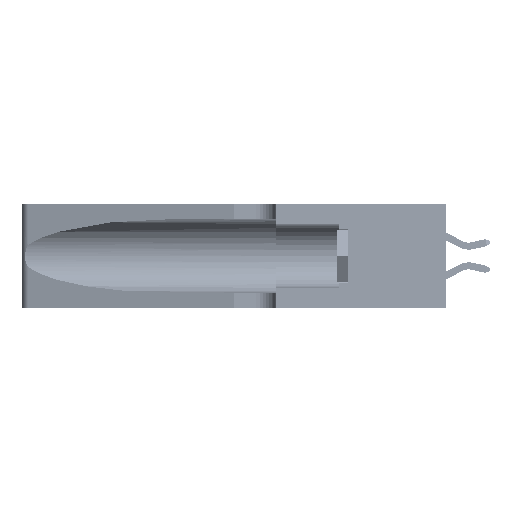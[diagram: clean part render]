
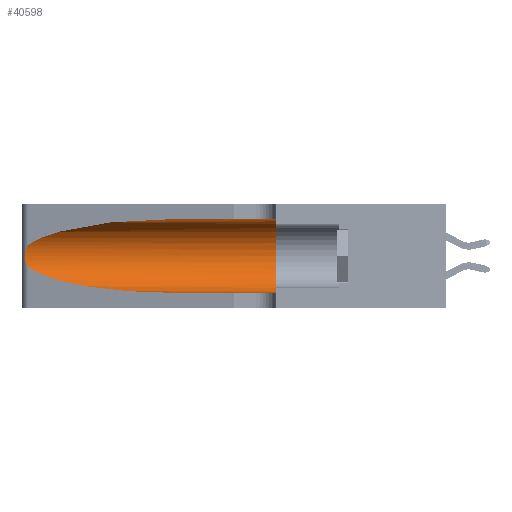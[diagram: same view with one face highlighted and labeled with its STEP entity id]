
A CAD part, left-side view. The second image highlights one B-rep face of the part: STEP entity #40598.
In plain terms, the highlighted cylindrical face has radius 3.308 mm (diameter 6.617 mm), a partial arc.
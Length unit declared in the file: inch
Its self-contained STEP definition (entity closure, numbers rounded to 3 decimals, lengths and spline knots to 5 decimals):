
#165 = CARTESIAN_POINT ( 'NONE',  ( 0.2373, 1.15595, 0.08982 ) ) ;
#395 = CARTESIAN_POINT ( 'NONE',  ( 0.1305, 1.61858, 0.185 ) ) ;
#1396 = CARTESIAN_POINT ( 'NONE',  ( 0.26018, 1.23835, 0.19895 ) ) ;
#1444 = ORIENTED_EDGE ( 'NONE', *, *, #46868, .T. ) ;
#2937 = ORIENTED_EDGE ( 'NONE', *, *, #30242, .T. ) ;
#3268 = DIRECTION ( 'NONE',  ( 0., 0., 1. ) ) ;
#3982 = CYLINDRICAL_SURFACE ( 'NONE', #19545, 0.13025 ) ;
#4039 = VECTOR ( 'NONE', #16669, 39.37008 ) ;
#4175 = CARTESIAN_POINT ( 'NONE',  ( 0.18966, 0.96281, 0.05475 ) ) ;
#4848 = CARTESIAN_POINT ( 'NONE',  ( 0.1305, 0.72297, 0.31525 ) ) ;
#5222 = FACE_OUTER_BOUND ( 'NONE', #39873, .T. ) ;
#5376 = CARTESIAN_POINT ( 'NONE',  ( 0.26075, 1.23896, 0.178 ) ) ;
#6524 = EDGE_CURVE ( 'NONE', #23491, #16954, #32752, .T. ) ;
#7786 = CARTESIAN_POINT ( 'NONE',  ( 0.1305, 0.35, 0.05475 ) ) ;
#8304 = DIRECTION ( 'NONE',  ( 0., 0., -1. ) ) ;
#8749 = CARTESIAN_POINT ( 'NONE',  ( 0.2373, 1.15595, 0.28018 ) ) ;
#9259 = CARTESIAN_POINT ( 'NONE',  ( 0.25856, 1.23593, 0.16098 ) ) ;
#10930 = VERTEX_POINT ( 'NONE', #28211 ) ;
#13111 = CARTESIAN_POINT ( 'NONE',  ( 0.25639, 1.23186, 0.15144 ) ) ;
#13795 = VERTEX_POINT ( 'NONE', #40203 ) ;
#14588 = CARTESIAN_POINT ( 'NONE',  ( 0.1305, 1.61858, 0.31525 ) ) ;
#16669 = DIRECTION ( 'NONE',  ( 0., -1., 0. ) ) ;
#16732 = CARTESIAN_POINT ( 'NONE',  ( 0.25487, 1.22718, 0.22369 ) ) ;
#16888 = CARTESIAN_POINT ( 'NONE',  ( 0.25487, 1.22718, 0.14631 ) ) ;
#16954 = VERTEX_POINT ( 'NONE', #48494 ) ;
#18870 = B_SPLINE_CURVE_WITH_KNOTS ( 'NONE', 3,
 ( #16732, #35430, #20499, #46677, #24292, #1396, #28073, #5376, #31846, #9259, #35581, #13111, #39286, #16888 ),
 .UNSPECIFIED., .F., .F.,
 ( 4, 2, 2, 2, 2, 2, 4 ),
 ( 0., 0.00027, 0.00053, 0.00107, 0.0016, 0.00187, 0.00214 ),
 .UNSPECIFIED. ) ;
#19545 = AXIS2_PLACEMENT_3D ( 'NONE', #395, #30924, #8304 ) ;
#20499 = CARTESIAN_POINT ( 'NONE',  ( 0.25639, 1.23184, 0.21858 ) ) ;
#21071 = EDGE_CURVE ( 'NONE', #10930, #13795, #48585, .T. ) ;
#22062 = CIRCLE ( 'NONE', #25625, 0.13025 ) ;
#22507 =( BOUNDED_CURVE ( )  B_SPLINE_CURVE ( 3, ( #4848, #27566, #8749, #35082 ),
 .UNSPECIFIED., .F., .T. ) 
 B_SPLINE_CURVE_WITH_KNOTS ( ( 4, 4 ),
 ( 1.5708, 2.84003 ),
 .UNSPECIFIED. ) 
 CURVE ( )  GEOMETRIC_REPRESENTATION_ITEM ( )  RATIONAL_B_SPLINE_CURVE ( ( 1., 0.87, 0.87, 1. ) ) 
 REPRESENTATION_ITEM ( '' )  );
#22757 = VECTOR ( 'NONE', #48307, 39.37008 ) ;
#23143 = CARTESIAN_POINT ( 'NONE',  ( 0.25487, 1.22718, 0.14631 ) ) ;
#23491 = VERTEX_POINT ( 'NONE', #43228 ) ;
#24292 = CARTESIAN_POINT ( 'NONE',  ( 0.25854, 1.2359, 0.20912 ) ) ;
#25625 = AXIS2_PLACEMENT_3D ( 'NONE', #48428, #26029, #3268 ) ;
#26029 = DIRECTION ( 'NONE',  ( 0., 1., 0. ) ) ;
#27566 = CARTESIAN_POINT ( 'NONE',  ( 0.18966, 0.96281, 0.31525 ) ) ;
#28073 = CARTESIAN_POINT ( 'NONE',  ( 0.26075, 1.23896, 0.19203 ) ) ;
#28211 = CARTESIAN_POINT ( 'NONE',  ( 0.25487, 1.22718, 0.14631 ) ) ;
#28576 = ORIENTED_EDGE ( 'NONE', *, *, #36854, .T. ) ;
#30242 = EDGE_CURVE ( 'NONE', #23491, #42915, #22507, .T. ) ;
#30719 = CARTESIAN_POINT ( 'NONE',  ( 0.1305, 0.72297, 0.05475 ) ) ;
#30924 = DIRECTION ( 'NONE',  ( 0., -1., 0. ) ) ;
#31126 = ORIENTED_EDGE ( 'NONE', *, *, #6524, .F. ) ;
#31192 = ORIENTED_EDGE ( 'NONE', *, *, #34451, .F. ) ;
#31846 = CARTESIAN_POINT ( 'NONE',  ( 0.26017, 1.23833, 0.17102 ) ) ;
#32752 = LINE ( 'NONE', #14588, #22757 ) ;
#34246 = LINE ( 'NONE', #42839, #4039 ) ;
#34451 = EDGE_CURVE ( 'NONE', #16954, #42503, #22062, .T. ) ;
#35082 = CARTESIAN_POINT ( 'NONE',  ( 0.25487, 1.22718, 0.22369 ) ) ;
#35430 = CARTESIAN_POINT ( 'NONE',  ( 0.25555, 1.22994, 0.2215 ) ) ;
#35581 = CARTESIAN_POINT ( 'NONE',  ( 0.25789, 1.23486, 0.15765 ) ) ;
#36425 = CARTESIAN_POINT ( 'NONE',  ( 0.25487, 1.22718, 0.22369 ) ) ;
#36854 = EDGE_CURVE ( 'NONE', #13795, #42503, #34246, .T. ) ;
#38516 = ORIENTED_EDGE ( 'NONE', *, *, #21071, .T. ) ;
#39286 = CARTESIAN_POINT ( 'NONE',  ( 0.25555, 1.22993, 0.14849 ) ) ;
#39873 = EDGE_LOOP ( 'NONE', ( #2937, #1444, #38516, #28576, #31192, #31126 ) ) ;
#40203 = CARTESIAN_POINT ( 'NONE',  ( 0.1305, 0.72297, 0.05475 ) ) ;
#40598 = ADVANCED_FACE ( 'NONE', ( #5222 ), #3982, .F. ) ;
#42503 = VERTEX_POINT ( 'NONE', #7786 ) ;
#42839 = CARTESIAN_POINT ( 'NONE',  ( 0.1305, 1.61858, 0.05475 ) ) ;
#42915 = VERTEX_POINT ( 'NONE', #36425 ) ;
#43228 = CARTESIAN_POINT ( 'NONE',  ( 0.1305, 0.72297, 0.31525 ) ) ;
#46677 = CARTESIAN_POINT ( 'NONE',  ( 0.25787, 1.23484, 0.2124 ) ) ;
#46868 = EDGE_CURVE ( 'NONE', #42915, #10930, #18870, .T. ) ;
#48307 = DIRECTION ( 'NONE',  ( 0., -1., 0. ) ) ;
#48428 = CARTESIAN_POINT ( 'NONE',  ( 0.1305, 0.35, 0.185 ) ) ;
#48494 = CARTESIAN_POINT ( 'NONE',  ( 0.1305, 0.35, 0.31525 ) ) ;
#48585 =( BOUNDED_CURVE ( )  B_SPLINE_CURVE ( 3, ( #23143, #165, #4175, #30719 ),
 .UNSPECIFIED., .F., .F. ) 
 B_SPLINE_CURVE_WITH_KNOTS ( ( 4, 4 ),
 ( 3.44316, 4.71239 ),
 .UNSPECIFIED. ) 
 CURVE ( )  GEOMETRIC_REPRESENTATION_ITEM ( )  RATIONAL_B_SPLINE_CURVE ( ( 1., 0.87, 0.87, 1. ) ) 
 REPRESENTATION_ITEM ( '' )  );
